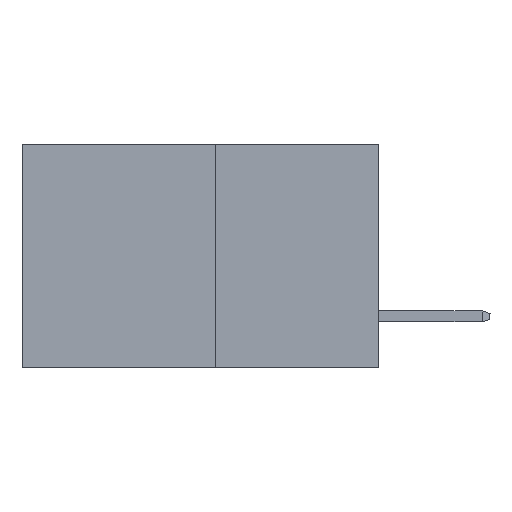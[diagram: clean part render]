
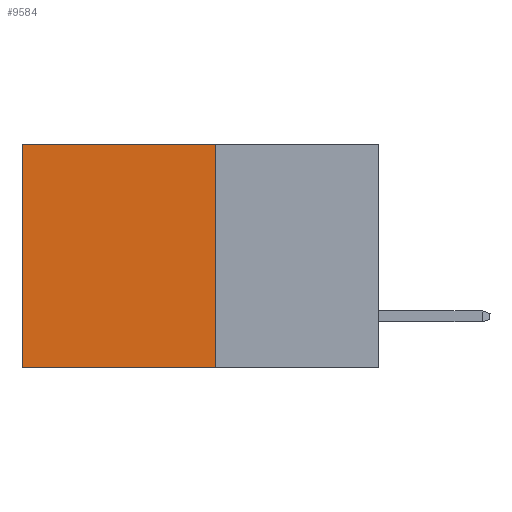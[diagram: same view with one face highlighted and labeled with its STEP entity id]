
A CAD part, left-side view. The second image highlights one B-rep face of the part: STEP entity #9584.
In plain terms, the highlighted planar face has unit normal (-1, 0, 0).
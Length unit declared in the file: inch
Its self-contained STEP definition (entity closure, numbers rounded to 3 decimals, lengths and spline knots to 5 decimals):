
#698 = EDGE_CURVE ( 'NONE', #11781, #3778, #10303, .T. ) ;
#1355 = VECTOR ( 'NONE', #3408, 39.37008 ) ;
#1544 = PLANE ( 'NONE',  #5693 ) ;
#2210 = EDGE_CURVE ( 'NONE', #12370, #8108, #5295, .T. ) ;
#2235 = ORIENTED_EDGE ( 'NONE', *, *, #7493, .T. ) ;
#2361 = ORIENTED_EDGE ( 'NONE', *, *, #2210, .F. ) ;
#2460 = ORIENTED_EDGE ( 'NONE', *, *, #8573, .F. ) ;
#2662 = DIRECTION ( 'NONE',  ( 0., 0., -1. ) ) ;
#2671 = CARTESIAN_POINT ( 'NONE',  ( 0.277, 0.59, -0.37 ) ) ;
#2685 = ORIENTED_EDGE ( 'NONE', *, *, #698, .T. ) ;
#3408 = DIRECTION ( 'NONE',  ( 0., 0., -1. ) ) ;
#3757 = CARTESIAN_POINT ( 'NONE',  ( 0.277, 0.59, -0.37 ) ) ;
#3778 = VERTEX_POINT ( 'NONE', #5436 ) ;
#3831 = DIRECTION ( 'NONE',  ( 0., 0., -1. ) ) ;
#4657 = VECTOR ( 'NONE', #13703, 39.37008 ) ;
#5295 = LINE ( 'NONE', #12726, #5646 ) ;
#5386 = EDGE_LOOP ( 'NONE', ( #2235, #2361, #2460, #2685 ) ) ;
#5436 = CARTESIAN_POINT ( 'NONE',  ( 0.277, 0.59, 0. ) ) ;
#5646 = VECTOR ( 'NONE', #13010, 39.37008 ) ;
#5693 = AXIS2_PLACEMENT_3D ( 'NONE', #7090, #9167, #2662 ) ;
#6099 = LINE ( 'NONE', #2671, #11316 ) ;
#6321 = CARTESIAN_POINT ( 'NONE',  ( 0.277, 0.27, -0.37 ) ) ;
#7090 = CARTESIAN_POINT ( 'NONE',  ( 0.277, 0.27, -0.37 ) ) ;
#7101 = CARTESIAN_POINT ( 'NONE',  ( 0.277, 0.27, 0. ) ) ;
#7493 = EDGE_CURVE ( 'NONE', #3778, #8108, #6099, .T. ) ;
#8108 = VERTEX_POINT ( 'NONE', #3757 ) ;
#8573 = EDGE_CURVE ( 'NONE', #11781, #12370, #10311, .T. ) ;
#9167 = DIRECTION ( 'NONE',  ( 1., 0., 0. ) ) ;
#9584 = ADVANCED_FACE ( 'NONE', ( #10922 ), #1544, .F. ) ;
#9612 = CARTESIAN_POINT ( 'NONE',  ( 0.277, 0.27, 0. ) ) ;
#9808 = CARTESIAN_POINT ( 'NONE',  ( 0.277, 0.27, -0.37 ) ) ;
#10303 = LINE ( 'NONE', #7101, #4657 ) ;
#10311 = LINE ( 'NONE', #9808, #1355 ) ;
#10922 = FACE_OUTER_BOUND ( 'NONE', #5386, .T. ) ;
#11316 = VECTOR ( 'NONE', #3831, 39.37008 ) ;
#11781 = VERTEX_POINT ( 'NONE', #9612 ) ;
#12370 = VERTEX_POINT ( 'NONE', #6321 ) ;
#12726 = CARTESIAN_POINT ( 'NONE',  ( 0.277, 0.27, -0.37 ) ) ;
#13010 = DIRECTION ( 'NONE',  ( 0., 1., 0. ) ) ;
#13703 = DIRECTION ( 'NONE',  ( 0., 1., 0. ) ) ;
